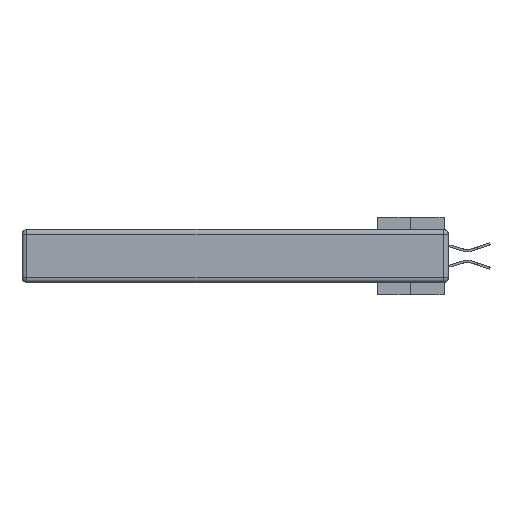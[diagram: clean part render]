
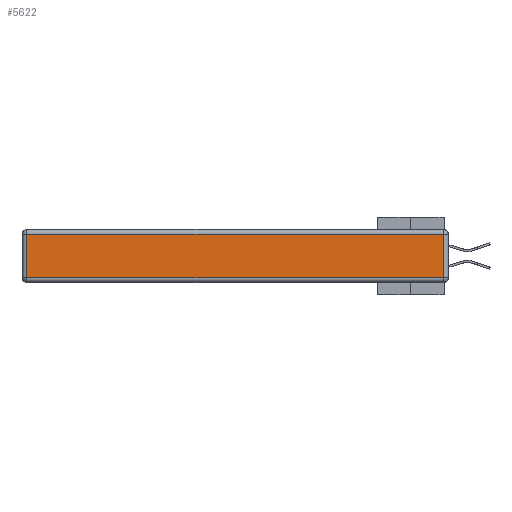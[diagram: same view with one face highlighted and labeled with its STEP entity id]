
A CAD part, left-side view. The second image highlights one B-rep face of the part: STEP entity #5622.
In plain terms, the highlighted planar face has unit normal (-1, 0, 0).
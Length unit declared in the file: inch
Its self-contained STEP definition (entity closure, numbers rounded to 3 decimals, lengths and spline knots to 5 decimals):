
#5622 = ADVANCED_FACE ( 'NONE', ( #23987 ), #21953, .T. ) ;
#8405 = DIRECTION ( 'NONE',  ( 0., 1., 0. ) ) ;
#8564 = CARTESIAN_POINT ( 'NONE',  ( 0., 2.75, -0.03 ) ) ;
#8777 = VECTOR ( 'NONE', #37156, 39.37008 ) ;
#9795 = ORIENTED_EDGE ( 'NONE', *, *, #10275, .T. ) ;
#9960 = EDGE_CURVE ( 'NONE', #26958, #34056, #35448, .T. ) ;
#10275 = EDGE_CURVE ( 'NONE', #32246, #26958, #44858, .T. ) ;
#10656 = CARTESIAN_POINT ( 'NONE',  ( 0., 0., -0.313 ) ) ;
#13514 = VERTEX_POINT ( 'NONE', #27297 ) ;
#14103 = DIRECTION ( 'NONE',  ( 0., -1., 0. ) ) ;
#14383 = DIRECTION ( 'NONE',  ( -1., 0., 0. ) ) ;
#20013 = VECTOR ( 'NONE', #8405, 39.37008 ) ;
#21426 = EDGE_CURVE ( 'NONE', #13514, #32246, #46199, .T. ) ;
#21953 = PLANE ( 'NONE',  #27279 ) ;
#22539 = LINE ( 'NONE', #29459, #27272 ) ;
#22583 = CARTESIAN_POINT ( 'NONE',  ( 0., 0.03, -0.313 ) ) ;
#23987 = FACE_OUTER_BOUND ( 'NONE', #41640, .T. ) ;
#24308 = CARTESIAN_POINT ( 'NONE',  ( 0., 0.03, -0.03 ) ) ;
#26958 = VERTEX_POINT ( 'NONE', #24308 ) ;
#27272 = VECTOR ( 'NONE', #48268, 39.37008 ) ;
#27279 = AXIS2_PLACEMENT_3D ( 'NONE', #29595, #14383, #36710 ) ;
#27297 = CARTESIAN_POINT ( 'NONE',  ( 0., 2.72, -0.313 ) ) ;
#27996 = ORIENTED_EDGE ( 'NONE', *, *, #48131, .T. ) ;
#29459 = CARTESIAN_POINT ( 'NONE',  ( 0., 2.72, -0.343 ) ) ;
#29595 = CARTESIAN_POINT ( 'NONE',  ( 0., 0., -0.343 ) ) ;
#32246 = VERTEX_POINT ( 'NONE', #22583 ) ;
#34056 = VERTEX_POINT ( 'NONE', #42734 ) ;
#35448 = LINE ( 'NONE', #8564, #20013 ) ;
#36710 = DIRECTION ( 'NONE',  ( 0., 0., 1. ) ) ;
#37156 = DIRECTION ( 'NONE',  ( 0., 0., 1. ) ) ;
#41099 = CARTESIAN_POINT ( 'NONE',  ( 0., 0.03, -0.343 ) ) ;
#41640 = EDGE_LOOP ( 'NONE', ( #45745, #9795, #41723, #27996 ) ) ;
#41723 = ORIENTED_EDGE ( 'NONE', *, *, #9960, .T. ) ;
#42638 = VECTOR ( 'NONE', #14103, 39.37008 ) ;
#42734 = CARTESIAN_POINT ( 'NONE',  ( 0., 2.72, -0.03 ) ) ;
#44858 = LINE ( 'NONE', #41099, #8777 ) ;
#45745 = ORIENTED_EDGE ( 'NONE', *, *, #21426, .T. ) ;
#46199 = LINE ( 'NONE', #10656, #42638 ) ;
#48131 = EDGE_CURVE ( 'NONE', #34056, #13514, #22539, .T. ) ;
#48268 = DIRECTION ( 'NONE',  ( 0., 0., -1. ) ) ;
